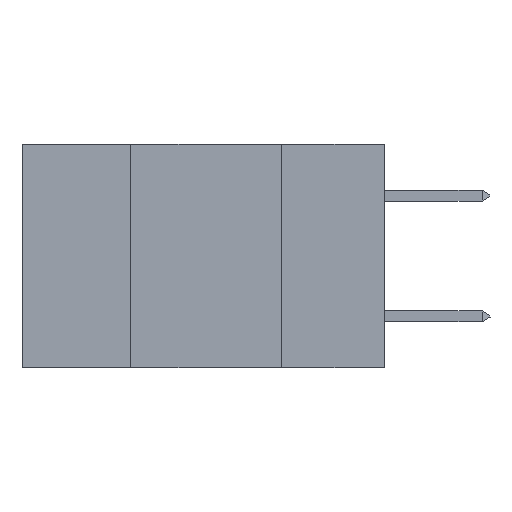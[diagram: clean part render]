
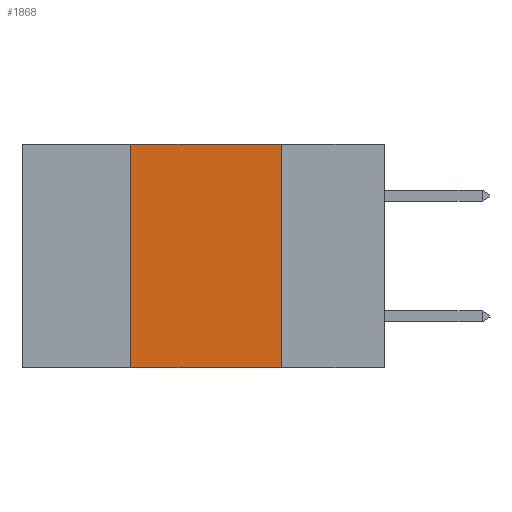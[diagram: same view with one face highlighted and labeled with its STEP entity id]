
A CAD part, left-side view. The second image highlights one B-rep face of the part: STEP entity #1868.
In plain terms, the highlighted planar face has unit normal (-1, 0, 0).
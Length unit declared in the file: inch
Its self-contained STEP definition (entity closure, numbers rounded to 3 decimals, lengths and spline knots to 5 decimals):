
#197 = EDGE_LOOP ( 'NONE', ( #16255, #408, #22862, #14840 ) ) ;
#408 = ORIENTED_EDGE ( 'NONE', *, *, #9909, .F. ) ;
#463 = VECTOR ( 'NONE', #18236, 39.37008 ) ;
#1597 = EDGE_CURVE ( 'NONE', #22325, #12812, #6086, .T. ) ;
#1868 = ADVANCED_FACE ( 'NONE', ( #8935 ), #17204, .F. ) ;
#2735 = CARTESIAN_POINT ( 'NONE',  ( 0., 0.17, 0. ) ) ;
#4782 = CARTESIAN_POINT ( 'NONE',  ( 0., 0.6, -0.37 ) ) ;
#4785 = CARTESIAN_POINT ( 'NONE',  ( 0., 0.42, 0. ) ) ;
#4827 = EDGE_CURVE ( 'NONE', #9484, #12812, #7627, .T. ) ;
#6086 = LINE ( 'NONE', #2735, #463 ) ;
#6349 = VECTOR ( 'NONE', #16496, 39.37008 ) ;
#7627 = LINE ( 'NONE', #4782, #15609 ) ;
#8935 = FACE_OUTER_BOUND ( 'NONE', #197, .T. ) ;
#9251 = EDGE_CURVE ( 'NONE', #9484, #15857, #11171, .T. ) ;
#9484 = VERTEX_POINT ( 'NONE', #10320 ) ;
#9909 = EDGE_CURVE ( 'NONE', #15857, #22325, #17446, .T. ) ;
#10320 = CARTESIAN_POINT ( 'NONE',  ( 0., 0.42, -0.37 ) ) ;
#11171 = LINE ( 'NONE', #4785, #13721 ) ;
#11941 = DIRECTION ( 'NONE',  ( 1., 0., 0. ) ) ;
#12812 = VERTEX_POINT ( 'NONE', #19413 ) ;
#13721 = VECTOR ( 'NONE', #19263, 39.37008 ) ;
#14840 = ORIENTED_EDGE ( 'NONE', *, *, #4827, .T. ) ;
#15609 = VECTOR ( 'NONE', #23270, 39.37008 ) ;
#15857 = VERTEX_POINT ( 'NONE', #22432 ) ;
#16255 = ORIENTED_EDGE ( 'NONE', *, *, #1597, .F. ) ;
#16496 = DIRECTION ( 'NONE',  ( 0., -1., 0. ) ) ;
#17204 = PLANE ( 'NONE',  #21483 ) ;
#17229 = CARTESIAN_POINT ( 'NONE',  ( 0., 0.17, 0. ) ) ;
#17446 = LINE ( 'NONE', #22230, #6349 ) ;
#18236 = DIRECTION ( 'NONE',  ( 0., 0., -1. ) ) ;
#18992 = DIRECTION ( 'NONE',  ( 0., 0., -1. ) ) ;
#19263 = DIRECTION ( 'NONE',  ( 0., 0., 1. ) ) ;
#19413 = CARTESIAN_POINT ( 'NONE',  ( 0., 0.17, -0.37 ) ) ;
#20930 = CARTESIAN_POINT ( 'NONE',  ( 0., 0.6, 0. ) ) ;
#21483 = AXIS2_PLACEMENT_3D ( 'NONE', #20930, #11941, #18992 ) ;
#22230 = CARTESIAN_POINT ( 'NONE',  ( 0., 0.6, 0. ) ) ;
#22325 = VERTEX_POINT ( 'NONE', #17229 ) ;
#22432 = CARTESIAN_POINT ( 'NONE',  ( 0., 0.42, 0. ) ) ;
#22862 = ORIENTED_EDGE ( 'NONE', *, *, #9251, .F. ) ;
#23270 = DIRECTION ( 'NONE',  ( 0., -1., 0. ) ) ;
